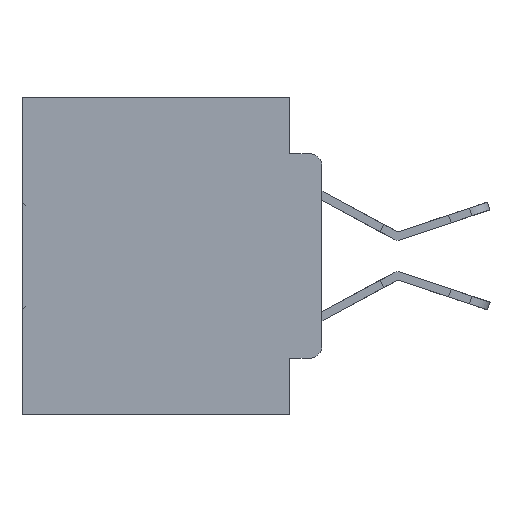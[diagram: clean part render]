
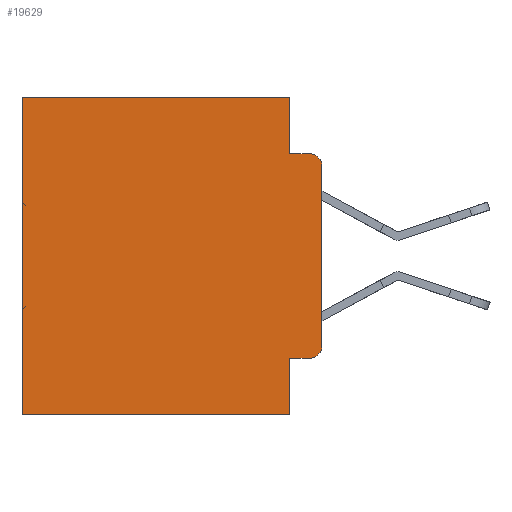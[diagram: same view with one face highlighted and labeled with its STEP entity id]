
A CAD part, left-side view. The second image highlights one B-rep face of the part: STEP entity #19629.
In plain terms, the highlighted planar face has unit normal (-1, 0, 0).
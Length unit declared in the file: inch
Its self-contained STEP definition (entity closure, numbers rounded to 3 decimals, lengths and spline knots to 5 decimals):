
#113 = EDGE_LOOP ( 'NONE', ( #29940, #14992, #23599, #13525, #8580, #3634, #6311, #23246, #20737, #13693 ) ) ;
#1201 = DIRECTION ( 'NONE',  ( 1., 0., 0. ) ) ;
#1808 = CARTESIAN_POINT ( 'NONE',  ( 0.298, 0.473, -0.5 ) ) ;
#3634 = ORIENTED_EDGE ( 'NONE', *, *, #9953, .T. ) ;
#3853 = VECTOR ( 'NONE', #14404, 39.37008 ) ;
#4909 = LINE ( 'NONE', #18693, #31006 ) ;
#4988 = CARTESIAN_POINT ( 'NONE',  ( 0.298, 0.473, 0. ) ) ;
#5748 = VERTEX_POINT ( 'NONE', #10304 ) ;
#6217 = VECTOR ( 'NONE', #10615, 39.37008 ) ;
#6311 = ORIENTED_EDGE ( 'NONE', *, *, #18767, .F. ) ;
#6790 = VECTOR ( 'NONE', #21472, 39.37008 ) ;
#7798 = VERTEX_POINT ( 'NONE', #31126 ) ;
#8580 = ORIENTED_EDGE ( 'NONE', *, *, #10613, .T. ) ;
#8913 = EDGE_CURVE ( 'NONE', #14156, #7798, #18012, .T. ) ;
#8984 = CARTESIAN_POINT ( 'NONE',  ( 0.298, 0., 0. ) ) ;
#9551 = EDGE_CURVE ( 'NONE', #11844, #10117, #16202, .T. ) ;
#9953 = EDGE_CURVE ( 'NONE', #24530, #31529, #10649, .T. ) ;
#10117 = VERTEX_POINT ( 'NONE', #16284 ) ;
#10189 = VECTOR ( 'NONE', #23684, 39.37008 ) ;
#10304 = CARTESIAN_POINT ( 'NONE',  ( 0.298, 0., -0.1085 ) ) ;
#10613 = EDGE_CURVE ( 'NONE', #14156, #24530, #24104, .T. ) ;
#10615 = DIRECTION ( 'NONE',  ( 0., -1., 0. ) ) ;
#10649 = LINE ( 'NONE', #26219, #6790 ) ;
#10745 = EDGE_CURVE ( 'NONE', #7798, #14623, #17287, .T. ) ;
#10981 = CARTESIAN_POINT ( 'NONE',  ( 0.298, 0., 0. ) ) ;
#11667 = FACE_OUTER_BOUND ( 'NONE', #113, .T. ) ;
#11844 = VERTEX_POINT ( 'NONE', #31510 ) ;
#11927 = LINE ( 'NONE', #8984, #14443 ) ;
#12846 = CARTESIAN_POINT ( 'NONE',  ( 0.298, 0.051, -0.0885 ) ) ;
#13114 = DIRECTION ( 'NONE',  ( 0., 0., -1. ) ) ;
#13525 = ORIENTED_EDGE ( 'NONE', *, *, #8913, .F. ) ;
#13693 = ORIENTED_EDGE ( 'NONE', *, *, #34467, .T. ) ;
#14156 = VERTEX_POINT ( 'NONE', #17895 ) ;
#14276 = EDGE_CURVE ( 'NONE', #5748, #14623, #31549, .T. ) ;
#14404 = DIRECTION ( 'NONE',  ( 0., 1., 0. ) ) ;
#14443 = VECTOR ( 'NONE', #19820, 39.37008 ) ;
#14623 = VERTEX_POINT ( 'NONE', #20295 ) ;
#14742 = EDGE_CURVE ( 'NONE', #11844, #30734, #4909, .T. ) ;
#14952 = DIRECTION ( 'NONE',  ( 0., 0., -1. ) ) ;
#14992 = ORIENTED_EDGE ( 'NONE', *, *, #14276, .T. ) ;
#15566 = DIRECTION ( 'NONE',  ( 0., 1., 0. ) ) ;
#16202 = LINE ( 'NONE', #24231, #6217 ) ;
#16284 = CARTESIAN_POINT ( 'NONE',  ( 0.298, 0.02, -0.4115 ) ) ;
#17287 = LINE ( 'NONE', #12846, #10189 ) ;
#17566 = CARTESIAN_POINT ( 'NONE',  ( 0.298, 0.02, -0.3915 ) ) ;
#17843 = DIRECTION ( 'NONE',  ( 0., 0., -1. ) ) ;
#17895 = CARTESIAN_POINT ( 'NONE',  ( 0.298, 0.051, 0. ) ) ;
#18012 = LINE ( 'NONE', #28693, #21800 ) ;
#18693 = CARTESIAN_POINT ( 'NONE',  ( 0.298, 0.051, 0. ) ) ;
#18767 = EDGE_CURVE ( 'NONE', #30734, #31529, #22082, .T. ) ;
#19629 = ADVANCED_FACE ( 'NONE', ( #11667 ), #27251, .F. ) ;
#19820 = DIRECTION ( 'NONE',  ( 0., 0., -1. ) ) ;
#20295 = CARTESIAN_POINT ( 'NONE',  ( 0.298, 0.02, -0.0885 ) ) ;
#20737 = ORIENTED_EDGE ( 'NONE', *, *, #9551, .T. ) ;
#21472 = DIRECTION ( 'NONE',  ( 0., 0., -1. ) ) ;
#21800 = VECTOR ( 'NONE', #17843, 39.37008 ) ;
#21914 = CIRCLE ( 'NONE', #31960, 0.02 ) ;
#22082 = LINE ( 'NONE', #27514, #3853 ) ;
#22805 = DIRECTION ( 'NONE',  ( -1., 0., 0. ) ) ;
#23246 = ORIENTED_EDGE ( 'NONE', *, *, #14742, .F. ) ;
#23599 = ORIENTED_EDGE ( 'NONE', *, *, #10745, .F. ) ;
#23684 = DIRECTION ( 'NONE',  ( 0., -1., 0. ) ) ;
#24104 = LINE ( 'NONE', #10981, #32485 ) ;
#24151 = DIRECTION ( 'NONE',  ( 0., 0., -1. ) ) ;
#24231 = CARTESIAN_POINT ( 'NONE',  ( 0.298, 0.051, -0.4115 ) ) ;
#24530 = VERTEX_POINT ( 'NONE', #4988 ) ;
#24691 = EDGE_CURVE ( 'NONE', #5748, #30231, #11927, .T. ) ;
#26219 = CARTESIAN_POINT ( 'NONE',  ( 0.298, 0.473, 0. ) ) ;
#26600 = DIRECTION ( 'NONE',  ( -1., 0., 0. ) ) ;
#26601 = CARTESIAN_POINT ( 'NONE',  ( 0.298, 0., -0.3915 ) ) ;
#27251 = PLANE ( 'NONE',  #27338 ) ;
#27338 = AXIS2_PLACEMENT_3D ( 'NONE', #33009, #1201, #29725 ) ;
#27514 = CARTESIAN_POINT ( 'NONE',  ( 0.298, 0., -0.5 ) ) ;
#28693 = CARTESIAN_POINT ( 'NONE',  ( 0.298, 0.051, 0. ) ) ;
#29725 = DIRECTION ( 'NONE',  ( 0., 0., -1. ) ) ;
#29940 = ORIENTED_EDGE ( 'NONE', *, *, #24691, .F. ) ;
#30231 = VERTEX_POINT ( 'NONE', #26601 ) ;
#30734 = VERTEX_POINT ( 'NONE', #32462 ) ;
#31006 = VECTOR ( 'NONE', #13114, 39.37008 ) ;
#31126 = CARTESIAN_POINT ( 'NONE',  ( 0.298, 0.051, -0.0885 ) ) ;
#31510 = CARTESIAN_POINT ( 'NONE',  ( 0.298, 0.051, -0.4115 ) ) ;
#31529 = VERTEX_POINT ( 'NONE', #1808 ) ;
#31549 = CIRCLE ( 'NONE', #34331, 0.02 ) ;
#31960 = AXIS2_PLACEMENT_3D ( 'NONE', #17566, #22805, #14952 ) ;
#32028 = CARTESIAN_POINT ( 'NONE',  ( 0.298, 0.02, -0.1085 ) ) ;
#32462 = CARTESIAN_POINT ( 'NONE',  ( 0.298, 0.051, -0.5 ) ) ;
#32485 = VECTOR ( 'NONE', #15566, 39.37008 ) ;
#33009 = CARTESIAN_POINT ( 'NONE',  ( 0.298, 0., 0. ) ) ;
#34331 = AXIS2_PLACEMENT_3D ( 'NONE', #32028, #26600, #24151 ) ;
#34467 = EDGE_CURVE ( 'NONE', #10117, #30231, #21914, .T. ) ;
